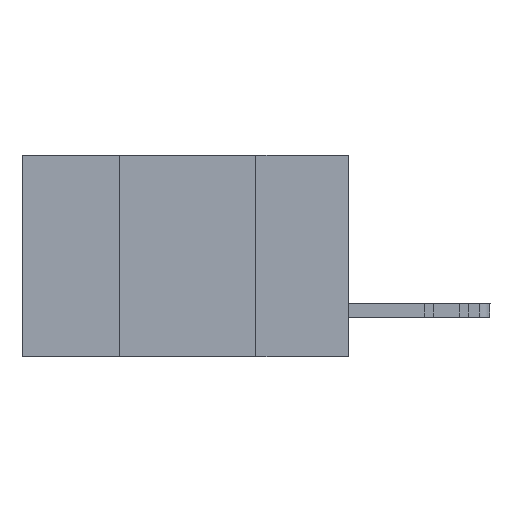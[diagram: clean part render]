
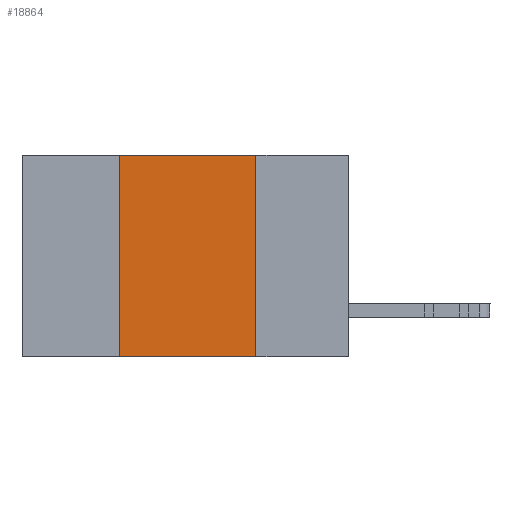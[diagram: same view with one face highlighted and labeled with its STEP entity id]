
A CAD part, left-side view. The second image highlights one B-rep face of the part: STEP entity #18864.
In plain terms, the highlighted planar face has unit normal (-1, 0, 0).
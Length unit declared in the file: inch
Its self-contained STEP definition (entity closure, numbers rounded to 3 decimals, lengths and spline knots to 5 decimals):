
#846 = VERTEX_POINT ( 'NONE', #3548 ) ;
#2376 = DIRECTION ( 'NONE',  ( 0., 0., 1. ) ) ;
#3548 = CARTESIAN_POINT ( 'NONE',  ( 0., 0.17, 0. ) ) ;
#3889 = VECTOR ( 'NONE', #20407, 39.37008 ) ;
#4071 = CARTESIAN_POINT ( 'NONE',  ( 0., 0.6, -0.37 ) ) ;
#4674 = EDGE_CURVE ( 'NONE', #19063, #21495, #7415, .T. ) ;
#4684 = EDGE_LOOP ( 'NONE', ( #12922, #11341, #14005, #7283 ) ) ;
#5503 = DIRECTION ( 'NONE',  ( 1., 0., 0. ) ) ;
#7283 = ORIENTED_EDGE ( 'NONE', *, *, #4674, .T. ) ;
#7415 = LINE ( 'NONE', #4071, #3889 ) ;
#9113 = AXIS2_PLACEMENT_3D ( 'NONE', #12652, #5503, #12536 ) ;
#9159 = CARTESIAN_POINT ( 'NONE',  ( 0., 0.6, 0. ) ) ;
#10367 = EDGE_CURVE ( 'NONE', #14982, #846, #21912, .T. ) ;
#11330 = CARTESIAN_POINT ( 'NONE',  ( 0., 0.42, -0.37 ) ) ;
#11341 = ORIENTED_EDGE ( 'NONE', *, *, #10367, .F. ) ;
#11666 = EDGE_CURVE ( 'NONE', #19063, #14982, #18456, .T. ) ;
#12536 = DIRECTION ( 'NONE',  ( 0., 0., -1. ) ) ;
#12652 = CARTESIAN_POINT ( 'NONE',  ( 0., 0.6, 0. ) ) ;
#12922 = ORIENTED_EDGE ( 'NONE', *, *, #22301, .F. ) ;
#12940 = CARTESIAN_POINT ( 'NONE',  ( 0., 0.17, -0.37 ) ) ;
#13214 = DIRECTION ( 'NONE',  ( 0., 0., -1. ) ) ;
#14005 = ORIENTED_EDGE ( 'NONE', *, *, #11666, .F. ) ;
#14475 = CARTESIAN_POINT ( 'NONE',  ( 0., 0.17, -0.37 ) ) ;
#14576 = PLANE ( 'NONE',  #9113 ) ;
#14982 = VERTEX_POINT ( 'NONE', #18749 ) ;
#17329 = VECTOR ( 'NONE', #18569, 39.37008 ) ;
#18456 = LINE ( 'NONE', #18698, #22319 ) ;
#18569 = DIRECTION ( 'NONE',  ( 0., -1., 0. ) ) ;
#18698 = CARTESIAN_POINT ( 'NONE',  ( 0., 0.42, -0.37 ) ) ;
#18749 = CARTESIAN_POINT ( 'NONE',  ( 0., 0.42, 0. ) ) ;
#18864 = ADVANCED_FACE ( 'NONE', ( #23574 ), #14576, .F. ) ;
#19063 = VERTEX_POINT ( 'NONE', #11330 ) ;
#19844 = VECTOR ( 'NONE', #13214, 39.37008 ) ;
#20407 = DIRECTION ( 'NONE',  ( 0., -1., 0. ) ) ;
#21495 = VERTEX_POINT ( 'NONE', #12940 ) ;
#21912 = LINE ( 'NONE', #9159, #17329 ) ;
#22301 = EDGE_CURVE ( 'NONE', #846, #21495, #23401, .T. ) ;
#22319 = VECTOR ( 'NONE', #2376, 39.37008 ) ;
#23401 = LINE ( 'NONE', #14475, #19844 ) ;
#23574 = FACE_OUTER_BOUND ( 'NONE', #4684, .T. ) ;
